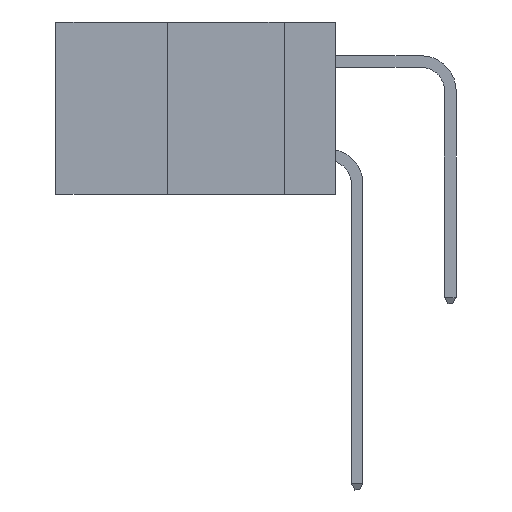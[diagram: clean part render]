
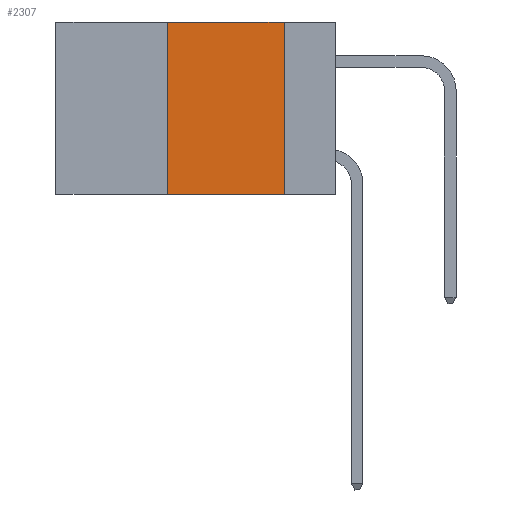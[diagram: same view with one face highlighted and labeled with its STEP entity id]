
A CAD part, left-side view. The second image highlights one B-rep face of the part: STEP entity #2307.
In plain terms, the highlighted planar face has unit normal (-1, 0, 0).
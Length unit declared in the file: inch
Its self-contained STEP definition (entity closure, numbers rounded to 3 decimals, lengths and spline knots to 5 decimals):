
#720 = VECTOR ( 'NONE', #12918, 39.37008 ) ;
#876 = LINE ( 'NONE', #3988, #10848 ) ;
#1288 = DIRECTION ( 'NONE',  ( 1., 0., 0. ) ) ;
#2030 = ORIENTED_EDGE ( 'NONE', *, *, #9527, .F. ) ;
#2307 = ADVANCED_FACE ( 'NONE', ( #5654 ), #3760, .F. ) ;
#2514 = LINE ( 'NONE', #2915, #16026 ) ;
#2710 = CARTESIAN_POINT ( 'NONE',  ( 0., 0.36, -0.37 ) ) ;
#2915 = CARTESIAN_POINT ( 'NONE',  ( 0., 0.6, 0. ) ) ;
#3336 = EDGE_CURVE ( 'NONE', #13628, #7452, #876, .T. ) ;
#3760 = PLANE ( 'NONE',  #10624 ) ;
#3809 = DIRECTION ( 'NONE',  ( 0., 0., 1. ) ) ;
#3850 = VERTEX_POINT ( 'NONE', #10558 ) ;
#3988 = CARTESIAN_POINT ( 'NONE',  ( 0., 0.36, 0. ) ) ;
#4368 = VECTOR ( 'NONE', #12216, 39.37008 ) ;
#4438 = ORIENTED_EDGE ( 'NONE', *, *, #14824, .T. ) ;
#4497 = EDGE_LOOP ( 'NONE', ( #6891, #2030, #7455, #4438 ) ) ;
#4672 = EDGE_CURVE ( 'NONE', #3850, #5233, #11183, .T. ) ;
#5233 = VERTEX_POINT ( 'NONE', #16188 ) ;
#5654 = FACE_OUTER_BOUND ( 'NONE', #4497, .T. ) ;
#6891 = ORIENTED_EDGE ( 'NONE', *, *, #4672, .F. ) ;
#7452 = VERTEX_POINT ( 'NONE', #15288 ) ;
#7455 = ORIENTED_EDGE ( 'NONE', *, *, #3336, .F. ) ;
#8435 = CARTESIAN_POINT ( 'NONE',  ( 0., 0.11, 0. ) ) ;
#9527 = EDGE_CURVE ( 'NONE', #7452, #3850, #2514, .T. ) ;
#10558 = CARTESIAN_POINT ( 'NONE',  ( 0., 0.11, 0. ) ) ;
#10624 = AXIS2_PLACEMENT_3D ( 'NONE', #11206, #1288, #13426 ) ;
#10848 = VECTOR ( 'NONE', #3809, 39.37008 ) ;
#11183 = LINE ( 'NONE', #8435, #4368 ) ;
#11206 = CARTESIAN_POINT ( 'NONE',  ( 0., 0.6, 0. ) ) ;
#11671 = CARTESIAN_POINT ( 'NONE',  ( 0., 0.6, -0.37 ) ) ;
#11891 = DIRECTION ( 'NONE',  ( 0., -1., 0. ) ) ;
#12216 = DIRECTION ( 'NONE',  ( 0., 0., -1. ) ) ;
#12918 = DIRECTION ( 'NONE',  ( 0., -1., 0. ) ) ;
#13426 = DIRECTION ( 'NONE',  ( 0., 0., -1. ) ) ;
#13628 = VERTEX_POINT ( 'NONE', #2710 ) ;
#14002 = LINE ( 'NONE', #11671, #720 ) ;
#14824 = EDGE_CURVE ( 'NONE', #13628, #5233, #14002, .T. ) ;
#15288 = CARTESIAN_POINT ( 'NONE',  ( 0., 0.36, 0. ) ) ;
#16026 = VECTOR ( 'NONE', #11891, 39.37008 ) ;
#16188 = CARTESIAN_POINT ( 'NONE',  ( 0., 0.11, -0.37 ) ) ;
